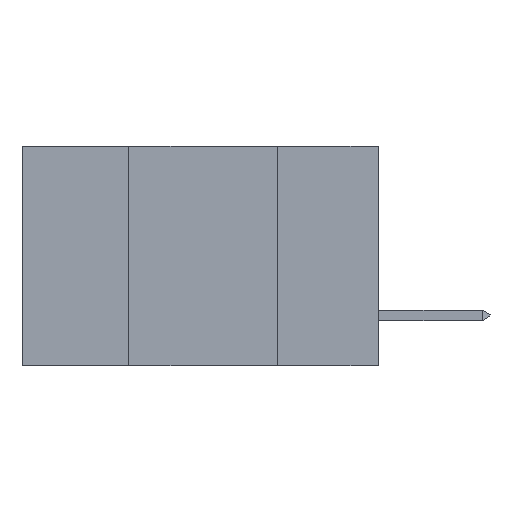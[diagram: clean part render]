
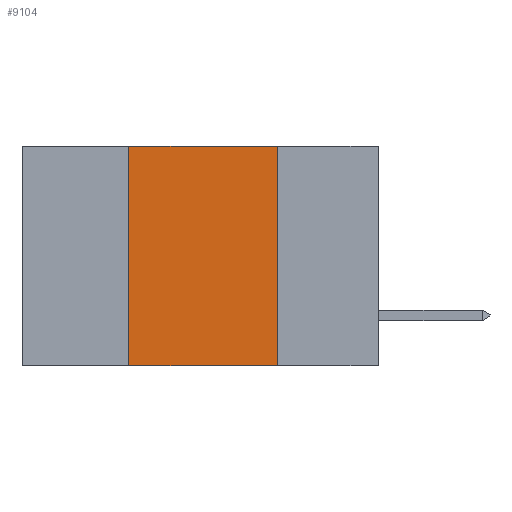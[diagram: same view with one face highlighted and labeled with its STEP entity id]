
A CAD part, left-side view. The second image highlights one B-rep face of the part: STEP entity #9104.
In plain terms, the highlighted planar face has unit normal (-1, 0, 0).
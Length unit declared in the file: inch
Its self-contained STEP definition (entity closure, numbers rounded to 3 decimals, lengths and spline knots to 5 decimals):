
#394 = CARTESIAN_POINT ( 'NONE',  ( 0., 0.6, 0. ) ) ;
#543 = EDGE_CURVE ( 'NONE', #12296, #4208, #860, .T. ) ;
#860 = LINE ( 'NONE', #6649, #12725 ) ;
#902 = VECTOR ( 'NONE', #13769, 39.37008 ) ;
#1432 = CARTESIAN_POINT ( 'NONE',  ( 0., 0.6, -0.37 ) ) ;
#2863 = DIRECTION ( 'NONE',  ( 0., 0., -1. ) ) ;
#3120 = EDGE_CURVE ( 'NONE', #12296, #8476, #11313, .T. ) ;
#4208 = VERTEX_POINT ( 'NONE', #5219 ) ;
#4430 = CARTESIAN_POINT ( 'NONE',  ( 0., 0.17, 0. ) ) ;
#4704 = ORIENTED_EDGE ( 'NONE', *, *, #3120, .T. ) ;
#5007 = FACE_OUTER_BOUND ( 'NONE', #12598, .T. ) ;
#5219 = CARTESIAN_POINT ( 'NONE',  ( 0., 0.42, 0. ) ) ;
#5402 = VECTOR ( 'NONE', #10644, 39.37008 ) ;
#5809 = VECTOR ( 'NONE', #6915, 39.37008 ) ;
#6649 = CARTESIAN_POINT ( 'NONE',  ( 0., 0.42, 0. ) ) ;
#6915 = DIRECTION ( 'NONE',  ( 0., 0., -1. ) ) ;
#7429 = EDGE_CURVE ( 'NONE', #13853, #8476, #12238, .T. ) ;
#7818 = EDGE_CURVE ( 'NONE', #4208, #13853, #10813, .T. ) ;
#8476 = VERTEX_POINT ( 'NONE', #14174 ) ;
#8509 = ORIENTED_EDGE ( 'NONE', *, *, #7818, .F. ) ;
#9028 = AXIS2_PLACEMENT_3D ( 'NONE', #394, #14258, #2863 ) ;
#9104 = ADVANCED_FACE ( 'NONE', ( #5007 ), #10815, .F. ) ;
#9319 = CARTESIAN_POINT ( 'NONE',  ( 0., 0.6, 0. ) ) ;
#10148 = DIRECTION ( 'NONE',  ( 0., 0., 1. ) ) ;
#10162 = CARTESIAN_POINT ( 'NONE',  ( 0., 0.17, 0. ) ) ;
#10644 = DIRECTION ( 'NONE',  ( 0., -1., 0. ) ) ;
#10813 = LINE ( 'NONE', #9319, #902 ) ;
#10815 = PLANE ( 'NONE',  #9028 ) ;
#10883 = CARTESIAN_POINT ( 'NONE',  ( 0., 0.42, -0.37 ) ) ;
#11313 = LINE ( 'NONE', #1432, #5402 ) ;
#11672 = ORIENTED_EDGE ( 'NONE', *, *, #7429, .F. ) ;
#12238 = LINE ( 'NONE', #10162, #5809 ) ;
#12296 = VERTEX_POINT ( 'NONE', #10883 ) ;
#12598 = EDGE_LOOP ( 'NONE', ( #11672, #8509, #13468, #4704 ) ) ;
#12725 = VECTOR ( 'NONE', #10148, 39.37008 ) ;
#13468 = ORIENTED_EDGE ( 'NONE', *, *, #543, .F. ) ;
#13769 = DIRECTION ( 'NONE',  ( 0., -1., 0. ) ) ;
#13853 = VERTEX_POINT ( 'NONE', #4430 ) ;
#14174 = CARTESIAN_POINT ( 'NONE',  ( 0., 0.17, -0.37 ) ) ;
#14258 = DIRECTION ( 'NONE',  ( 1., 0., 0. ) ) ;
